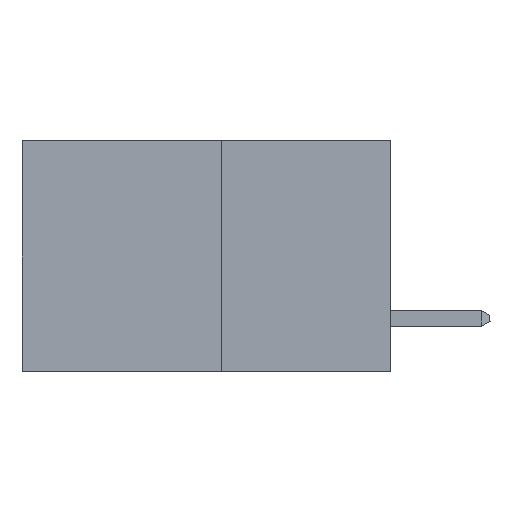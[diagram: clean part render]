
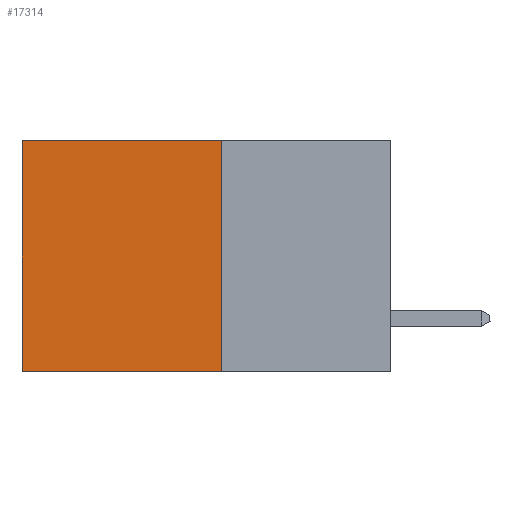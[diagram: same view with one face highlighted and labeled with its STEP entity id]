
A CAD part, left-side view. The second image highlights one B-rep face of the part: STEP entity #17314.
In plain terms, the highlighted planar face has unit normal (-1, 0, 0).
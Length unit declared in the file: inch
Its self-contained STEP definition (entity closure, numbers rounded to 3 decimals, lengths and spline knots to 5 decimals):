
#399 = LINE ( 'NONE', #3801, #11498 ) ;
#521 = CARTESIAN_POINT ( 'NONE',  ( 0.277, 0.27, -0.37 ) ) ;
#834 = CARTESIAN_POINT ( 'NONE',  ( 0.277, 0.59, 0. ) ) ;
#1137 = LINE ( 'NONE', #6263, #4552 ) ;
#1382 = ORIENTED_EDGE ( 'NONE', *, *, #4259, .T. ) ;
#2017 = DIRECTION ( 'NONE',  ( 0., 0., -1. ) ) ;
#2021 = EDGE_CURVE ( 'NONE', #12471, #11656, #8266, .T. ) ;
#3755 = LINE ( 'NONE', #7753, #14314 ) ;
#3801 = CARTESIAN_POINT ( 'NONE',  ( 0.277, 0.27, -0.37 ) ) ;
#4259 = EDGE_CURVE ( 'NONE', #12471, #4369, #3755, .T. ) ;
#4293 = VECTOR ( 'NONE', #8935, 39.37008 ) ;
#4369 = VERTEX_POINT ( 'NONE', #834 ) ;
#4552 = VECTOR ( 'NONE', #16328, 39.37008 ) ;
#4571 = ORIENTED_EDGE ( 'NONE', *, *, #2021, .F. ) ;
#4904 = CARTESIAN_POINT ( 'NONE',  ( 0.277, 0.27, -0.37 ) ) ;
#6145 = CARTESIAN_POINT ( 'NONE',  ( 0.277, 0.59, -0.37 ) ) ;
#6244 = EDGE_CURVE ( 'NONE', #4369, #10730, #1137, .T. ) ;
#6263 = CARTESIAN_POINT ( 'NONE',  ( 0.277, 0.59, -0.37 ) ) ;
#7753 = CARTESIAN_POINT ( 'NONE',  ( 0.277, 0.27, 0. ) ) ;
#7852 = ORIENTED_EDGE ( 'NONE', *, *, #13200, .F. ) ;
#8266 = LINE ( 'NONE', #9565, #4293 ) ;
#8935 = DIRECTION ( 'NONE',  ( 0., 0., -1. ) ) ;
#9565 = CARTESIAN_POINT ( 'NONE',  ( 0.277, 0.27, -0.37 ) ) ;
#10532 = ORIENTED_EDGE ( 'NONE', *, *, #6244, .T. ) ;
#10626 = DIRECTION ( 'NONE',  ( 1., 0., 0. ) ) ;
#10730 = VERTEX_POINT ( 'NONE', #6145 ) ;
#11498 = VECTOR ( 'NONE', #16695, 39.37008 ) ;
#11656 = VERTEX_POINT ( 'NONE', #4904 ) ;
#12471 = VERTEX_POINT ( 'NONE', #15263 ) ;
#13200 = EDGE_CURVE ( 'NONE', #11656, #10730, #399, .T. ) ;
#14314 = VECTOR ( 'NONE', #14962, 39.37008 ) ;
#14962 = DIRECTION ( 'NONE',  ( 0., 1., 0. ) ) ;
#15146 = EDGE_LOOP ( 'NONE', ( #10532, #7852, #4571, #1382 ) ) ;
#15263 = CARTESIAN_POINT ( 'NONE',  ( 0.277, 0.27, 0. ) ) ;
#16325 = PLANE ( 'NONE',  #18130 ) ;
#16328 = DIRECTION ( 'NONE',  ( 0., 0., -1. ) ) ;
#16695 = DIRECTION ( 'NONE',  ( 0., 1., 0. ) ) ;
#17314 = ADVANCED_FACE ( 'NONE', ( #17555 ), #16325, .F. ) ;
#17555 = FACE_OUTER_BOUND ( 'NONE', #15146, .T. ) ;
#18130 = AXIS2_PLACEMENT_3D ( 'NONE', #521, #10626, #2017 ) ;
